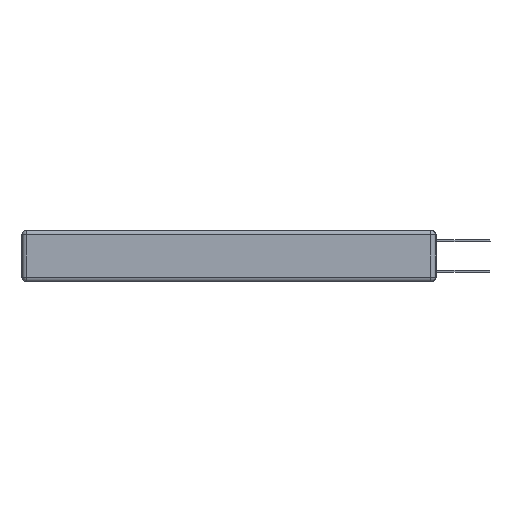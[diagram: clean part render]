
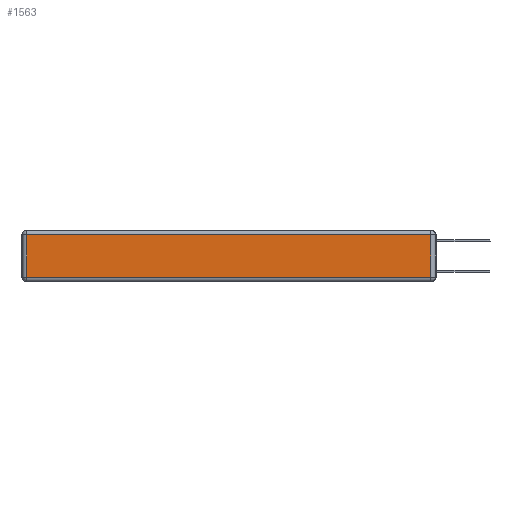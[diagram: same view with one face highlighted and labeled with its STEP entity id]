
A CAD part, left-side view. The second image highlights one B-rep face of the part: STEP entity #1563.
In plain terms, the highlighted planar face has unit normal (-1, 0, 0).
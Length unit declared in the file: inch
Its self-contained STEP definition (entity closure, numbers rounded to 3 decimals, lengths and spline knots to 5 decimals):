
#233 = FACE_OUTER_BOUND ( 'NONE', #10644, .T. ) ;
#1338 = DIRECTION ( 'NONE',  ( 0., -1., 0. ) ) ;
#1563 = ADVANCED_FACE ( 'NONE', ( #233 ), #19542, .T. ) ;
#3291 = LINE ( 'NONE', #15747, #7523 ) ;
#4102 = VECTOR ( 'NONE', #1338, 39.37008 ) ;
#5322 = CARTESIAN_POINT ( 'NONE',  ( 0., 0.03, -0.03 ) ) ;
#5327 = LINE ( 'NONE', #18422, #10526 ) ;
#5702 = CARTESIAN_POINT ( 'NONE',  ( 0., 0.03, -0.313 ) ) ;
#6459 = EDGE_CURVE ( 'NONE', #17482, #23297, #10291, .T. ) ;
#6730 = DIRECTION ( 'NONE',  ( 0., 0., 1. ) ) ;
#7057 = CARTESIAN_POINT ( 'NONE',  ( 0., 2.72, -0.313 ) ) ;
#7523 = VECTOR ( 'NONE', #9652, 39.37008 ) ;
#7598 = AXIS2_PLACEMENT_3D ( 'NONE', #15151, #19272, #6730 ) ;
#7823 = VERTEX_POINT ( 'NONE', #5322 ) ;
#8038 = EDGE_CURVE ( 'NONE', #15165, #17482, #5327, .T. ) ;
#9652 = DIRECTION ( 'NONE',  ( 0., 0., 1. ) ) ;
#9937 = VECTOR ( 'NONE', #12323, 39.37008 ) ;
#10291 = LINE ( 'NONE', #13805, #4102 ) ;
#10526 = VECTOR ( 'NONE', #22456, 39.37008 ) ;
#10644 = EDGE_LOOP ( 'NONE', ( #12541, #25379, #20196, #16856 ) ) ;
#12323 = DIRECTION ( 'NONE',  ( 0., 1., 0. ) ) ;
#12541 = ORIENTED_EDGE ( 'NONE', *, *, #6459, .T. ) ;
#13805 = CARTESIAN_POINT ( 'NONE',  ( 0., 0., -0.313 ) ) ;
#13913 = EDGE_CURVE ( 'NONE', #7823, #15165, #23674, .T. ) ;
#15151 = CARTESIAN_POINT ( 'NONE',  ( 0., 0., -0.343 ) ) ;
#15165 = VERTEX_POINT ( 'NONE', #18995 ) ;
#15747 = CARTESIAN_POINT ( 'NONE',  ( 0., 0.03, -0.343 ) ) ;
#16544 = EDGE_CURVE ( 'NONE', #23297, #7823, #3291, .T. ) ;
#16856 = ORIENTED_EDGE ( 'NONE', *, *, #8038, .T. ) ;
#17482 = VERTEX_POINT ( 'NONE', #7057 ) ;
#18422 = CARTESIAN_POINT ( 'NONE',  ( 0., 2.72, -0.343 ) ) ;
#18995 = CARTESIAN_POINT ( 'NONE',  ( 0., 2.72, -0.03 ) ) ;
#19272 = DIRECTION ( 'NONE',  ( -1., 0., 0. ) ) ;
#19542 = PLANE ( 'NONE',  #7598 ) ;
#20196 = ORIENTED_EDGE ( 'NONE', *, *, #13913, .T. ) ;
#22456 = DIRECTION ( 'NONE',  ( 0., 0., -1. ) ) ;
#23297 = VERTEX_POINT ( 'NONE', #5702 ) ;
#23674 = LINE ( 'NONE', #24884, #9937 ) ;
#24884 = CARTESIAN_POINT ( 'NONE',  ( 0., 2.75, -0.03 ) ) ;
#25379 = ORIENTED_EDGE ( 'NONE', *, *, #16544, .T. ) ;
